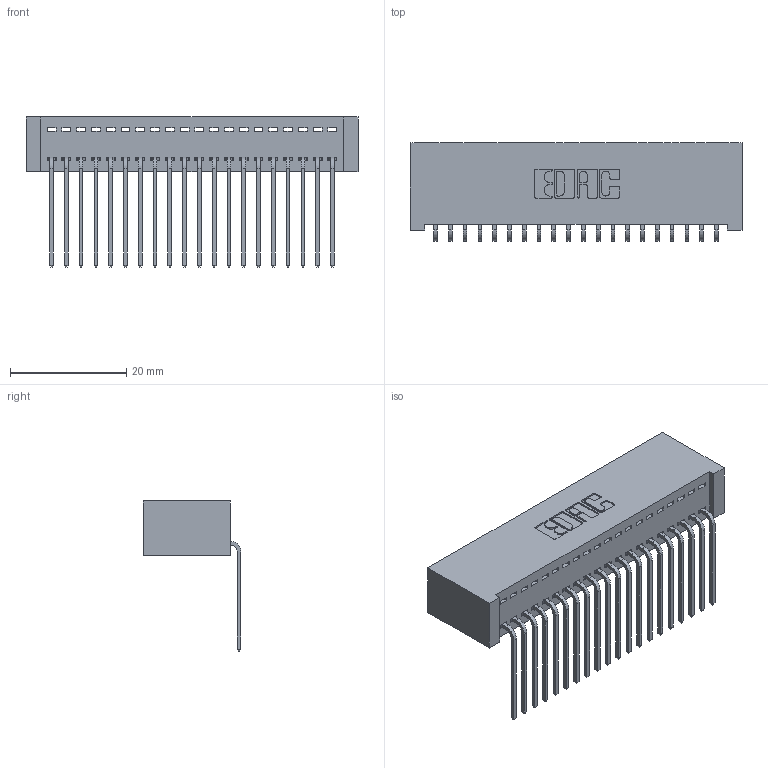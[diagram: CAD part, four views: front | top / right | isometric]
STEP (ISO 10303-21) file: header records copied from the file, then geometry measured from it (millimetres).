
FILE_DESCRIPTION (( 'STEP AP203' ), '1' );
FILE_NAME ('342-020-559-101.STEP', '2019-10-01T21:31:36', ( '' ), ( '' ), 'SwSTEP 2.0', 'SolidWorks 2016', '' );
FILE_SCHEMA (( 'CONFIG_CONTROL_DESIGN' ));
Length unit declared in the file: inch
Products named in the file (3): 342 Part_Lugless; 345-292-001_558 559 Tail - 1; 342-020-559-101
Assembly tree (21 placements, depth 2):
  342-020-559-101
    342 Part_Lugless
    345-292-001_558 559 Tail - 1  x20
Bounding box: 57.05 x 16.83 x 25.78 mm (x, y, z)
Volume: 5396.6 mm3; surface area: 8215.6 mm2
Topology: 21 solids, 21 shells, 1302 faces, 3915 edges, 2582 vertices
Faces by surface type: plane 942, cylinder 360
Entity records: 14747 total; most frequent: CARTESIAN_POINT 2554, ORIENTED_EDGE 2510, DIRECTION 2191, EDGE_CURVE 1255, LINE 1135, VECTOR 1135, VERTEX_POINT 834, AXIS2_PLACEMENT_3D 528
